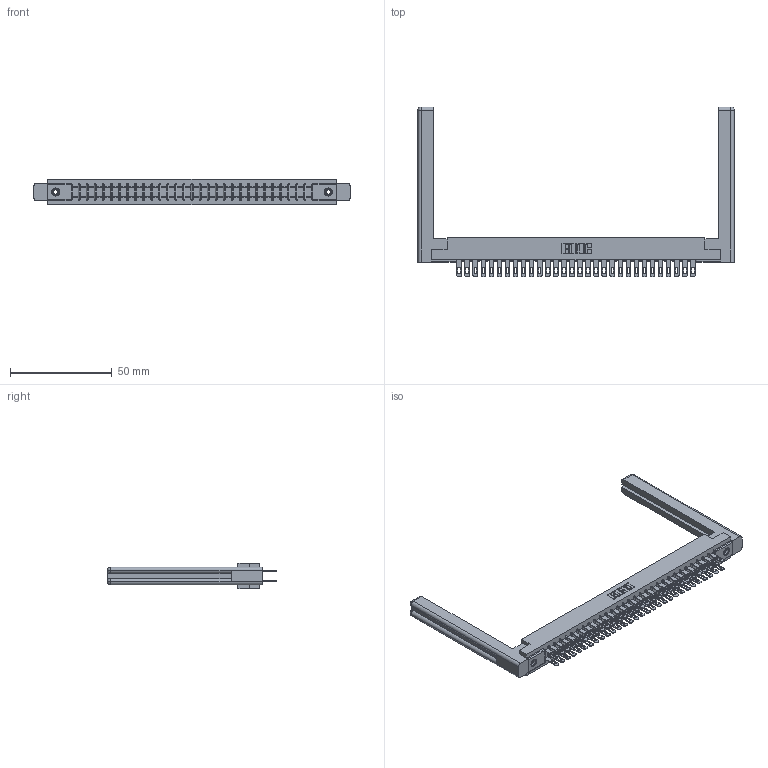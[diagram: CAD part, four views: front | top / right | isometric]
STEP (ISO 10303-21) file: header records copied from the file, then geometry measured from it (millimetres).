
FILE_DESCRIPTION (( 'STEP AP203' ), '1' );
FILE_NAME ('307-060-400-258.STEP', '2020-09-30T13:31:44', ( '' ), ( '' ), 'SwSTEP 2.0', 'SolidWorks 2020', '' );
FILE_SCHEMA (( 'CONFIG_CONTROL_DESIGN' ));
Length unit declared in the file: inch
Products named in the file (5): 307-060-400-258; 345-250-001_345-250-001-102; 307-220-058; 307-290-001_500; 307 Part_.156 Dia Mounting Holes
Assembly tree (65 placements, depth 2):
  307-060-400-258
    307 Part_.156 Dia Mounting Holes
    307-290-001_500  x60
    307-220-058  x2
    345-250-001_345-250-001-102  x2
Bounding box: 155.5 x 83.49 x 12.7 mm (x, y, z)
Volume: 23751.7 mm3; surface area: 25944.5 mm2
Topology: 65 solids, 65 shells, 3051 faces, 8477 edges, 5474 vertices
Faces by surface type: plane 1954, cylinder 1011, sphere 62, torus 12, cone 12
Entity records: 30765 total; most frequent: CARTESIAN_POINT 5053, ORIENTED_EDGE 4948, DIRECTION 4914, EDGE_CURVE 2474, LINE 1888, VECTOR 1888, VERTEX_POINT 1598, AXIS2_PLACEMENT_3D 1513
